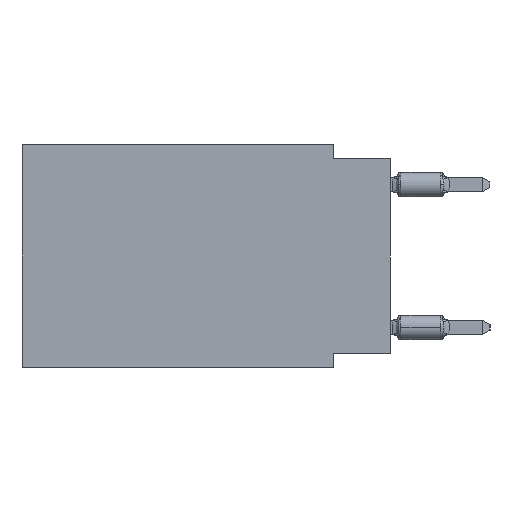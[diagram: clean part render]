
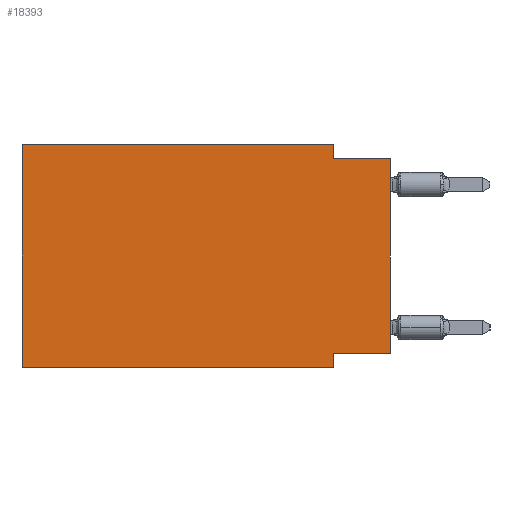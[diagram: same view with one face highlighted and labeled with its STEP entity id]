
A CAD part, left-side view. The second image highlights one B-rep face of the part: STEP entity #18393.
In plain terms, the highlighted planar face has unit normal (-1, 0, 0).
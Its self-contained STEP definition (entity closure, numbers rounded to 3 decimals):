
#1095 = DIRECTION ( 'NONE',  ( 0., 0., -1. ) ) ;
#1102 = VERTEX_POINT ( 'NONE', #8041 ) ;
#1200 = CARTESIAN_POINT ( 'NONE',  ( 0., 0., -9.271 ) ) ;
#1355 = VECTOR ( 'NONE', #1095, 1000. ) ;
#1383 = VECTOR ( 'NONE', #34333, 1000. ) ;
#2172 = VECTOR ( 'NONE', #16714, 1000. ) ;
#2531 = VERTEX_POINT ( 'NONE', #15217 ) ;
#2565 = EDGE_CURVE ( 'NONE', #15993, #2531, #2630, .T. ) ;
#2630 = LINE ( 'NONE', #6004, #8842 ) ;
#2946 = CARTESIAN_POINT ( 'NONE',  ( 0., 0., -9.271 ) ) ;
#3058 = EDGE_CURVE ( 'NONE', #30899, #31322, #6542, .T. ) ;
#3109 = LINE ( 'NONE', #6889, #1383 ) ;
#3151 = DIRECTION ( 'NONE',  ( 0., -1., 0. ) ) ;
#3288 = CARTESIAN_POINT ( 'NONE',  ( 0., 16.383, 0. ) ) ;
#3553 = DIRECTION ( 'NONE',  ( 0., -1., 0. ) ) ;
#4300 = CARTESIAN_POINT ( 'NONE',  ( 0., 16.383, 0. ) ) ;
#4529 = LINE ( 'NONE', #10734, #2172 ) ;
#5745 = CARTESIAN_POINT ( 'NONE',  ( 0., 0., 0. ) ) ;
#6004 = CARTESIAN_POINT ( 'NONE',  ( 0., 0., -0.635 ) ) ;
#6243 = CARTESIAN_POINT ( 'NONE',  ( 0., 2.54, -9.271 ) ) ;
#6542 = LINE ( 'NONE', #18744, #36351 ) ;
#6558 = CARTESIAN_POINT ( 'NONE',  ( 0., 16.383, -9.906 ) ) ;
#6619 = ORIENTED_EDGE ( 'NONE', *, *, #34473, .F. ) ;
#6889 = CARTESIAN_POINT ( 'NONE',  ( 0., 16.383, 0. ) ) ;
#7307 = EDGE_LOOP ( 'NONE', ( #9129, #11298, #23004, #11776, #32670, #35759, #15545, #6619 ) ) ;
#8031 = VECTOR ( 'NONE', #3151, 1000. ) ;
#8041 = CARTESIAN_POINT ( 'NONE',  ( 0., 2.54, -9.906 ) ) ;
#8842 = VECTOR ( 'NONE', #12022, 1000. ) ;
#9129 = ORIENTED_EDGE ( 'NONE', *, *, #14297, .T. ) ;
#9291 = CARTESIAN_POINT ( 'NONE',  ( 0., 2.54, -0.635 ) ) ;
#10699 = DIRECTION ( 'NONE',  ( 1., 0., 0. ) ) ;
#10734 = CARTESIAN_POINT ( 'NONE',  ( 0., 2.54, 0. ) ) ;
#11298 = ORIENTED_EDGE ( 'NONE', *, *, #2565, .F. ) ;
#11560 = DIRECTION ( 'NONE',  ( 0., 0., 1. ) ) ;
#11776 = ORIENTED_EDGE ( 'NONE', *, *, #3058, .F. ) ;
#12022 = DIRECTION ( 'NONE',  ( 0., -1., 0. ) ) ;
#13273 = VERTEX_POINT ( 'NONE', #6243 ) ;
#14297 = EDGE_CURVE ( 'NONE', #37461, #2531, #15144, .T. ) ;
#15144 = LINE ( 'NONE', #5745, #20129 ) ;
#15217 = CARTESIAN_POINT ( 'NONE',  ( 0., 0., -0.635 ) ) ;
#15545 = ORIENTED_EDGE ( 'NONE', *, *, #17675, .F. ) ;
#15828 = EDGE_CURVE ( 'NONE', #31322, #15993, #4529, .T. ) ;
#15993 = VERTEX_POINT ( 'NONE', #9291 ) ;
#15999 = DIRECTION ( 'NONE',  ( 0., 1., 0. ) ) ;
#16688 = CARTESIAN_POINT ( 'NONE',  ( 0., 2.54, -9.906 ) ) ;
#16714 = DIRECTION ( 'NONE',  ( 0., 0., -1. ) ) ;
#17675 = EDGE_CURVE ( 'NONE', #13273, #1102, #28512, .T. ) ;
#18255 = EDGE_CURVE ( 'NONE', #35882, #30899, #3109, .T. ) ;
#18393 = ADVANCED_FACE ( 'NONE', ( #18891 ), #31131, .F. ) ;
#18744 = CARTESIAN_POINT ( 'NONE',  ( 0., 16.383, 0. ) ) ;
#18891 = FACE_OUTER_BOUND ( 'NONE', #7307, .T. ) ;
#20129 = VECTOR ( 'NONE', #11560, 1000. ) ;
#22821 = LINE ( 'NONE', #1200, #24023 ) ;
#23004 = ORIENTED_EDGE ( 'NONE', *, *, #15828, .F. ) ;
#24023 = VECTOR ( 'NONE', #15999, 1000. ) ;
#25462 = EDGE_CURVE ( 'NONE', #35882, #1102, #36788, .T. ) ;
#27273 = CARTESIAN_POINT ( 'NONE',  ( 0., 2.54, 0. ) ) ;
#27954 = CARTESIAN_POINT ( 'NONE',  ( 0., 16.383, -9.906 ) ) ;
#28512 = LINE ( 'NONE', #16688, #1355 ) ;
#30899 = VERTEX_POINT ( 'NONE', #3288 ) ;
#31131 = PLANE ( 'NONE',  #33963 ) ;
#31322 = VERTEX_POINT ( 'NONE', #27273 ) ;
#32119 = DIRECTION ( 'NONE',  ( 0., 0., -1. ) ) ;
#32670 = ORIENTED_EDGE ( 'NONE', *, *, #18255, .F. ) ;
#33963 = AXIS2_PLACEMENT_3D ( 'NONE', #4300, #10699, #32119 ) ;
#34333 = DIRECTION ( 'NONE',  ( 0., 0., 1. ) ) ;
#34473 = EDGE_CURVE ( 'NONE', #37461, #13273, #22821, .T. ) ;
#35759 = ORIENTED_EDGE ( 'NONE', *, *, #25462, .T. ) ;
#35882 = VERTEX_POINT ( 'NONE', #6558 ) ;
#36351 = VECTOR ( 'NONE', #3553, 1000. ) ;
#36788 = LINE ( 'NONE', #27954, #8031 ) ;
#37461 = VERTEX_POINT ( 'NONE', #2946 ) ;
